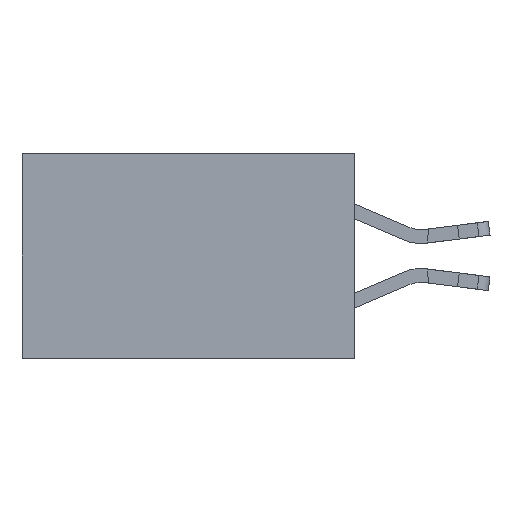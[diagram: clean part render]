
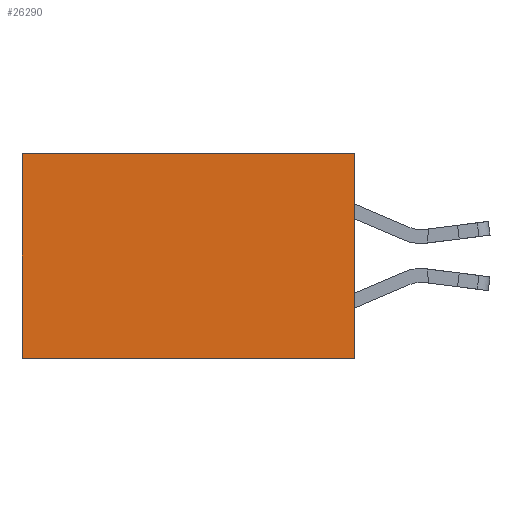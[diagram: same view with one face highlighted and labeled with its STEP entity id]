
A CAD part, left-side view. The second image highlights one B-rep face of the part: STEP entity #26290.
In plain terms, the highlighted planar face has unit normal (-1, 0, 0).
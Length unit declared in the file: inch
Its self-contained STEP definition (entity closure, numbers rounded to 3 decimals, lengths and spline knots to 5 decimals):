
#1375 = VECTOR ( 'NONE', #25231, 39.37008 ) ;
#2088 = CARTESIAN_POINT ( 'NONE',  ( 0.298, 0., 0. ) ) ;
#3629 = VERTEX_POINT ( 'NONE', #26914 ) ;
#5397 = DIRECTION ( 'NONE',  ( 0., 1., 0. ) ) ;
#5628 = EDGE_CURVE ( 'NONE', #3629, #15025, #7718, .T. ) ;
#6591 = CARTESIAN_POINT ( 'NONE',  ( 0.298, 0., -0.37 ) ) ;
#6820 = DIRECTION ( 'NONE',  ( 1., 0., 0. ) ) ;
#7128 = AXIS2_PLACEMENT_3D ( 'NONE', #20477, #6820, #22735 ) ;
#7718 = LINE ( 'NONE', #10487, #18432 ) ;
#9487 = CARTESIAN_POINT ( 'NONE',  ( 0.298, 0., -0.37 ) ) ;
#9646 = VECTOR ( 'NONE', #5397, 39.37008 ) ;
#10487 = CARTESIAN_POINT ( 'NONE',  ( 0.298, 0.6, 0. ) ) ;
#12149 = CARTESIAN_POINT ( 'NONE',  ( 0.298, 0., 0. ) ) ;
#13590 = EDGE_CURVE ( 'NONE', #23222, #3629, #21799, .T. ) ;
#13638 = PLANE ( 'NONE',  #7128 ) ;
#14534 = EDGE_CURVE ( 'NONE', #23222, #27342, #24207, .T. ) ;
#15025 = VERTEX_POINT ( 'NONE', #20497 ) ;
#16217 = CARTESIAN_POINT ( 'NONE',  ( 0.298, 0., 0. ) ) ;
#16456 = EDGE_LOOP ( 'NONE', ( #17594, #20942, #27359, #20147 ) ) ;
#17594 = ORIENTED_EDGE ( 'NONE', *, *, #5628, .T. ) ;
#18432 = VECTOR ( 'NONE', #23610, 39.37008 ) ;
#20147 = ORIENTED_EDGE ( 'NONE', *, *, #13590, .T. ) ;
#20477 = CARTESIAN_POINT ( 'NONE',  ( 0.298, 0., 0. ) ) ;
#20497 = CARTESIAN_POINT ( 'NONE',  ( 0.298, 0.6, -0.37 ) ) ;
#20942 = ORIENTED_EDGE ( 'NONE', *, *, #24420, .F. ) ;
#21799 = LINE ( 'NONE', #12149, #9646 ) ;
#21965 = LINE ( 'NONE', #9487, #26505 ) ;
#22735 = DIRECTION ( 'NONE',  ( 0., 0., -1. ) ) ;
#23222 = VERTEX_POINT ( 'NONE', #2088 ) ;
#23610 = DIRECTION ( 'NONE',  ( 0., 0., -1. ) ) ;
#24207 = LINE ( 'NONE', #16217, #1375 ) ;
#24420 = EDGE_CURVE ( 'NONE', #27342, #15025, #21965, .T. ) ;
#25231 = DIRECTION ( 'NONE',  ( 0., 0., -1. ) ) ;
#25257 = FACE_OUTER_BOUND ( 'NONE', #16456, .T. ) ;
#26290 = ADVANCED_FACE ( 'NONE', ( #25257 ), #13638, .F. ) ;
#26505 = VECTOR ( 'NONE', #27617, 39.37008 ) ;
#26914 = CARTESIAN_POINT ( 'NONE',  ( 0.298, 0.6, 0. ) ) ;
#27342 = VERTEX_POINT ( 'NONE', #6591 ) ;
#27359 = ORIENTED_EDGE ( 'NONE', *, *, #14534, .F. ) ;
#27617 = DIRECTION ( 'NONE',  ( 0., 1., 0. ) ) ;
